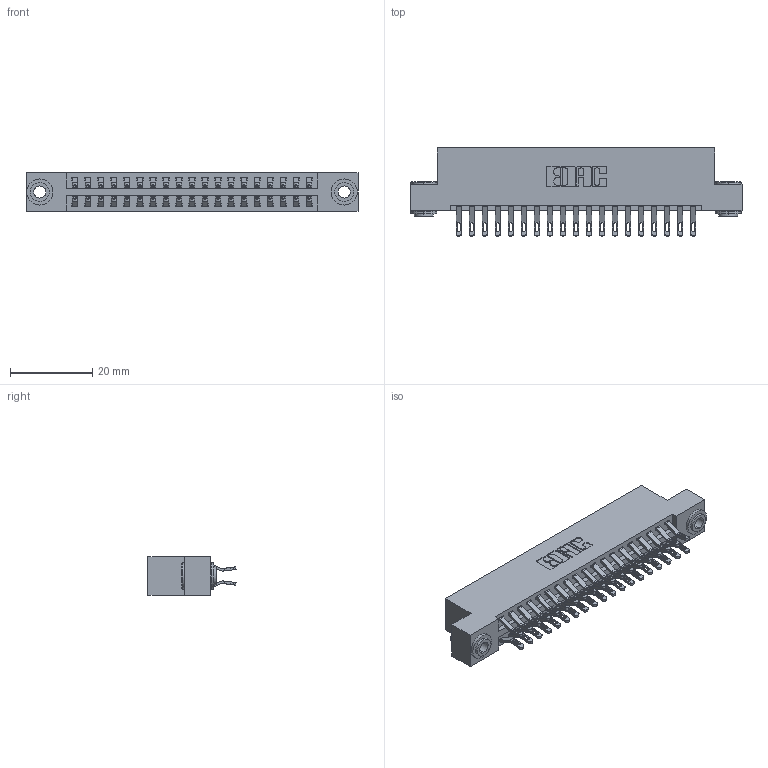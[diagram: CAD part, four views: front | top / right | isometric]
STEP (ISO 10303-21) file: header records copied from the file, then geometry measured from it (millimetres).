
FILE_DESCRIPTION (( 'STEP AP203' ), '1' );
FILE_NAME ('396-038-555-203.STEP', '2018-09-06T08:43:49', ( '' ), ( '' ), 'SwSTEP 2.0', 'SolidWorks 2016', '' );
FILE_SCHEMA (( 'CONFIG_CONTROL_DESIGN' ));
Length unit declared in the file: inch
Products named in the file (4): 346 Part_Flush Mounting Lugs - 0.156 Dia-TH; 345-292-001_555 Tail; 345-250-002_345-250-002-102; 396-038-555-203
Assembly tree (41 placements, depth 2):
  396-038-555-203
    346 Part_Flush Mounting Lugs - 0.156 Dia-TH
    345-292-001_555 Tail  x38
    345-250-002_345-250-002-102  x2
Bounding box: 80.9 x 21.46 x 9.4 mm (x, y, z)
Volume: 7839.6 mm3; surface area: 11021.7 mm2
Topology: 41 solids, 41 shells, 2364 faces, 7359 edges, 4902 vertices
Faces by surface type: plane 1340, cylinder 1016, cone 8
Entity records: 16472 total; most frequent: CARTESIAN_POINT 2757, ORIENTED_EDGE 2654, DIRECTION 2481, EDGE_CURVE 1327, VECTOR 1075, LINE 1075, VERTEX_POINT 882, AXIS2_PLACEMENT_3D 703
